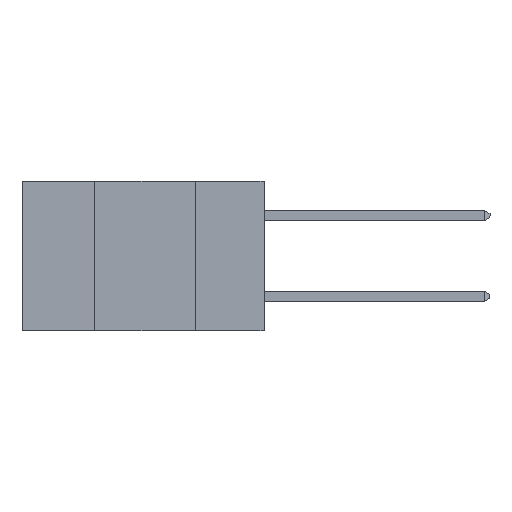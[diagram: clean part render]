
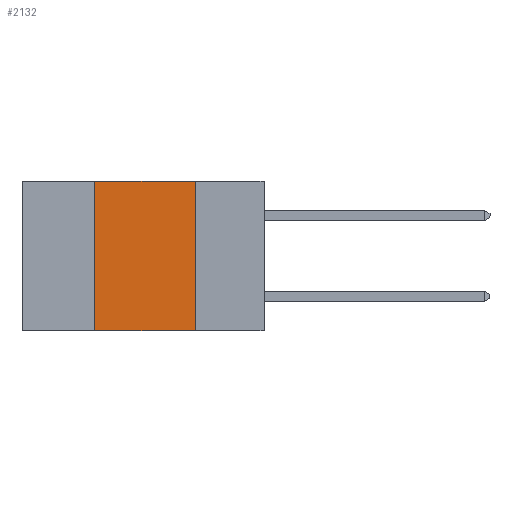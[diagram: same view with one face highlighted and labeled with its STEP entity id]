
A CAD part, left-side view. The second image highlights one B-rep face of the part: STEP entity #2132.
In plain terms, the highlighted planar face has unit normal (-1, 0, 0).
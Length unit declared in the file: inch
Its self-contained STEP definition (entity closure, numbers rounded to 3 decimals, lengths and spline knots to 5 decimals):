
#66 = LINE ( 'NONE', #10733, #8007 ) ;
#328 = AXIS2_PLACEMENT_3D ( 'NONE', #6790, #7742, #1873 ) ;
#365 = LINE ( 'NONE', #11492, #10768 ) ;
#669 = EDGE_CURVE ( 'NONE', #2245, #3082, #365, .T. ) ;
#792 = PLANE ( 'NONE',  #328 ) ;
#1231 = CARTESIAN_POINT ( 'NONE',  ( 0., 0.42, -0.37 ) ) ;
#1374 = CARTESIAN_POINT ( 'NONE',  ( 0., 0.17, 0. ) ) ;
#1384 = ORIENTED_EDGE ( 'NONE', *, *, #8055, .F. ) ;
#1873 = DIRECTION ( 'NONE',  ( 0., 0., -1. ) ) ;
#2132 = ADVANCED_FACE ( 'NONE', ( #6934 ), #792, .F. ) ;
#2245 = VERTEX_POINT ( 'NONE', #4994 ) ;
#2319 = DIRECTION ( 'NONE',  ( 0., 0., 1. ) ) ;
#2348 = LINE ( 'NONE', #9125, #9194 ) ;
#2666 = ORIENTED_EDGE ( 'NONE', *, *, #669, .F. ) ;
#2977 = VERTEX_POINT ( 'NONE', #1231 ) ;
#3021 = ORIENTED_EDGE ( 'NONE', *, *, #7442, .F. ) ;
#3082 = VERTEX_POINT ( 'NONE', #1374 ) ;
#3159 = VERTEX_POINT ( 'NONE', #4509 ) ;
#4061 = ORIENTED_EDGE ( 'NONE', *, *, #6789, .T. ) ;
#4495 = VECTOR ( 'NONE', #5236, 39.37008 ) ;
#4509 = CARTESIAN_POINT ( 'NONE',  ( 0., 0.17, -0.37 ) ) ;
#4663 = EDGE_LOOP ( 'NONE', ( #1384, #2666, #3021, #4061 ) ) ;
#4994 = CARTESIAN_POINT ( 'NONE',  ( 0., 0.42, 0. ) ) ;
#5029 = DIRECTION ( 'NONE',  ( 0., -1., 0. ) ) ;
#5236 = DIRECTION ( 'NONE',  ( 0., 0., -1. ) ) ;
#6789 = EDGE_CURVE ( 'NONE', #2977, #3159, #66, .T. ) ;
#6790 = CARTESIAN_POINT ( 'NONE',  ( 0., 0.6, 0. ) ) ;
#6934 = FACE_OUTER_BOUND ( 'NONE', #4663, .T. ) ;
#7442 = EDGE_CURVE ( 'NONE', #2977, #2245, #2348, .T. ) ;
#7742 = DIRECTION ( 'NONE',  ( 1., 0., 0. ) ) ;
#8007 = VECTOR ( 'NONE', #5029, 39.37008 ) ;
#8055 = EDGE_CURVE ( 'NONE', #3082, #3159, #11792, .T. ) ;
#9125 = CARTESIAN_POINT ( 'NONE',  ( 0., 0.42, 0. ) ) ;
#9194 = VECTOR ( 'NONE', #2319, 39.37008 ) ;
#10733 = CARTESIAN_POINT ( 'NONE',  ( 0., 0.6, -0.37 ) ) ;
#10768 = VECTOR ( 'NONE', #11488, 39.37008 ) ;
#11488 = DIRECTION ( 'NONE',  ( 0., -1., 0. ) ) ;
#11492 = CARTESIAN_POINT ( 'NONE',  ( 0., 0.6, 0. ) ) ;
#11792 = LINE ( 'NONE', #11873, #4495 ) ;
#11873 = CARTESIAN_POINT ( 'NONE',  ( 0., 0.17, 0. ) ) ;
